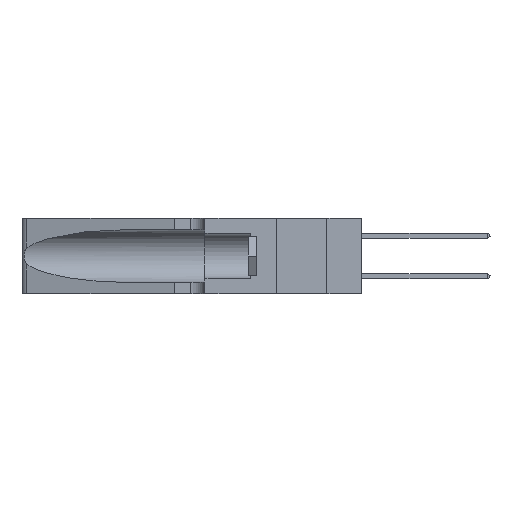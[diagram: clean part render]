
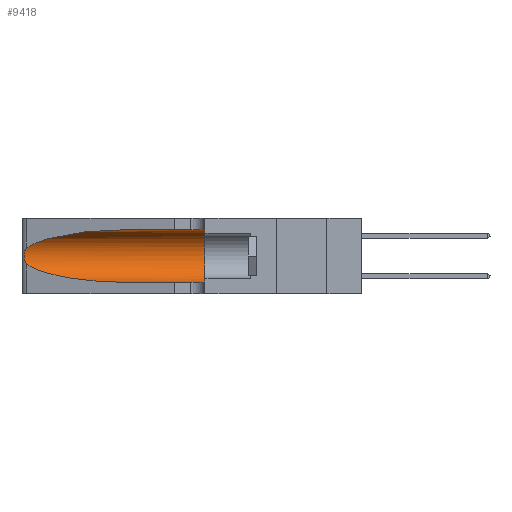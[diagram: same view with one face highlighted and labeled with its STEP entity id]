
A CAD part, left-side view. The second image highlights one B-rep face of the part: STEP entity #9418.
In plain terms, the highlighted cylindrical face has radius 3.308 mm (diameter 6.617 mm), a partial arc.
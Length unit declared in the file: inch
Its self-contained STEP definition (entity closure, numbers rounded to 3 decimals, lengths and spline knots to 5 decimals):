
#87 = LINE ( 'NONE', #23511, #12327 ) ;
#203 =( BOUNDED_CURVE ( )  B_SPLINE_CURVE ( 3, ( #25161, #13648, #16006, #1521 ),
 .UNSPECIFIED., .F., .F. ) 
 B_SPLINE_CURVE_WITH_KNOTS ( ( 4, 4 ),
 ( 3.44316, 4.71239 ),
 .UNSPECIFIED. ) 
 CURVE ( )  GEOMETRIC_REPRESENTATION_ITEM ( )  RATIONAL_B_SPLINE_CURVE ( ( 1., 0.87, 0.87, 1. ) ) 
 REPRESENTATION_ITEM ( '' )  );
#208 = CARTESIAN_POINT ( 'NONE',  ( 0.1305, 0.35, 0.31525 ) ) ;
#245 = CARTESIAN_POINT ( 'NONE',  ( 0.1305, 0.72297, 0.31525 ) ) ;
#1023 = CARTESIAN_POINT ( 'NONE',  ( 0.1305, 0.35, 0.185 ) ) ;
#1088 = CARTESIAN_POINT ( 'NONE',  ( 0.25787, 1.23484, 0.2124 ) ) ;
#1180 = B_SPLINE_CURVE_WITH_KNOTS ( 'NONE', 3,
 ( #27204, #29515, #15594, #1088, #17959, #3569, #20283, #6040, #22623, #8475, #24944, #10955, #27307, #13334 ),
 .UNSPECIFIED., .F., .F.,
 ( 4, 2, 2, 2, 2, 2, 4 ),
 ( 0., 0.00027, 0.00053, 0.00107, 0.0016, 0.00187, 0.00214 ),
 .UNSPECIFIED. ) ;
#1521 = CARTESIAN_POINT ( 'NONE',  ( 0.1305, 0.72297, 0.05475 ) ) ;
#1813 = EDGE_CURVE ( 'NONE', #19770, #26988, #3550, .T. ) ;
#2785 = ORIENTED_EDGE ( 'NONE', *, *, #14595, .T. ) ;
#3497 = DIRECTION ( 'NONE',  ( 0., 0., 1. ) ) ;
#3550 =( BOUNDED_CURVE ( )  B_SPLINE_CURVE ( 3, ( #245, #28720, #7532, #17137 ),
 .UNSPECIFIED., .F., .F. ) 
 B_SPLINE_CURVE_WITH_KNOTS ( ( 4, 4 ),
 ( 1.5708, 2.84003 ),
 .UNSPECIFIED. ) 
 CURVE ( )  GEOMETRIC_REPRESENTATION_ITEM ( )  RATIONAL_B_SPLINE_CURVE ( ( 1., 0.87, 0.87, 1. ) ) 
 REPRESENTATION_ITEM ( '' )  );
#3569 = CARTESIAN_POINT ( 'NONE',  ( 0.26018, 1.23835, 0.19895 ) ) ;
#3670 = EDGE_CURVE ( 'NONE', #19770, #26783, #16084, .T. ) ;
#5677 = CARTESIAN_POINT ( 'NONE',  ( 0.25487, 1.22718, 0.22369 ) ) ;
#6040 = CARTESIAN_POINT ( 'NONE',  ( 0.26075, 1.23896, 0.178 ) ) ;
#7050 = ORIENTED_EDGE ( 'NONE', *, *, #1813, .T. ) ;
#7532 = CARTESIAN_POINT ( 'NONE',  ( 0.2373, 1.15595, 0.28018 ) ) ;
#7551 = EDGE_CURVE ( 'NONE', #8156, #12607, #87, .T. ) ;
#8156 = VERTEX_POINT ( 'NONE', #30273 ) ;
#8475 = CARTESIAN_POINT ( 'NONE',  ( 0.25856, 1.23593, 0.16098 ) ) ;
#9418 = ADVANCED_FACE ( 'NONE', ( #23163 ), #22436, .F. ) ;
#9447 = DIRECTION ( 'NONE',  ( 0., -1., 0. ) ) ;
#9835 = ORIENTED_EDGE ( 'NONE', *, *, #19317, .T. ) ;
#10521 = VECTOR ( 'NONE', #18555, 39.37008 ) ;
#10955 = CARTESIAN_POINT ( 'NONE',  ( 0.25639, 1.23186, 0.15144 ) ) ;
#11575 = CARTESIAN_POINT ( 'NONE',  ( 0.1305, 1.61858, 0.185 ) ) ;
#11638 = CARTESIAN_POINT ( 'NONE',  ( 0.1305, 0.35, 0.05475 ) ) ;
#11726 = ORIENTED_EDGE ( 'NONE', *, *, #13005, .F. ) ;
#12327 = VECTOR ( 'NONE', #9447, 39.37008 ) ;
#12607 = VERTEX_POINT ( 'NONE', #11638 ) ;
#13005 = EDGE_CURVE ( 'NONE', #26783, #12607, #24573, .T. ) ;
#13021 = AXIS2_PLACEMENT_3D ( 'NONE', #1023, #17888, #3497 ) ;
#13334 = CARTESIAN_POINT ( 'NONE',  ( 0.25487, 1.22718, 0.14631 ) ) ;
#13648 = CARTESIAN_POINT ( 'NONE',  ( 0.2373, 1.15595, 0.08982 ) ) ;
#14595 = EDGE_CURVE ( 'NONE', #26988, #21667, #1180, .T. ) ;
#14648 = ORIENTED_EDGE ( 'NONE', *, *, #7551, .T. ) ;
#15192 = ORIENTED_EDGE ( 'NONE', *, *, #3670, .F. ) ;
#15594 = CARTESIAN_POINT ( 'NONE',  ( 0.25639, 1.23184, 0.21858 ) ) ;
#16006 = CARTESIAN_POINT ( 'NONE',  ( 0.18966, 0.96281, 0.05475 ) ) ;
#16084 = LINE ( 'NONE', #16227, #10521 ) ;
#16227 = CARTESIAN_POINT ( 'NONE',  ( 0.1305, 1.61858, 0.31525 ) ) ;
#16307 = DIRECTION ( 'NONE',  ( 0., -1., 0. ) ) ;
#17137 = CARTESIAN_POINT ( 'NONE',  ( 0.25487, 1.22718, 0.22369 ) ) ;
#17888 = DIRECTION ( 'NONE',  ( 0., 1., 0. ) ) ;
#17959 = CARTESIAN_POINT ( 'NONE',  ( 0.25854, 1.2359, 0.20912 ) ) ;
#18123 = AXIS2_PLACEMENT_3D ( 'NONE', #11575, #16307, #23222 ) ;
#18555 = DIRECTION ( 'NONE',  ( 0., -1., 0. ) ) ;
#19317 = EDGE_CURVE ( 'NONE', #21667, #8156, #203, .T. ) ;
#19770 = VERTEX_POINT ( 'NONE', #21535 ) ;
#20283 = CARTESIAN_POINT ( 'NONE',  ( 0.26075, 1.23896, 0.19203 ) ) ;
#21535 = CARTESIAN_POINT ( 'NONE',  ( 0.1305, 0.72297, 0.31525 ) ) ;
#21667 = VERTEX_POINT ( 'NONE', #28671 ) ;
#22436 = CYLINDRICAL_SURFACE ( 'NONE', #18123, 0.13025 ) ;
#22623 = CARTESIAN_POINT ( 'NONE',  ( 0.26017, 1.23833, 0.17102 ) ) ;
#23163 = FACE_OUTER_BOUND ( 'NONE', #26831, .T. ) ;
#23222 = DIRECTION ( 'NONE',  ( 0., 0., -1. ) ) ;
#23511 = CARTESIAN_POINT ( 'NONE',  ( 0.1305, 1.61858, 0.05475 ) ) ;
#24573 = CIRCLE ( 'NONE', #13021, 0.13025 ) ;
#24944 = CARTESIAN_POINT ( 'NONE',  ( 0.25789, 1.23486, 0.15765 ) ) ;
#25161 = CARTESIAN_POINT ( 'NONE',  ( 0.25487, 1.22718, 0.14631 ) ) ;
#26783 = VERTEX_POINT ( 'NONE', #208 ) ;
#26831 = EDGE_LOOP ( 'NONE', ( #7050, #2785, #9835, #14648, #11726, #15192 ) ) ;
#26988 = VERTEX_POINT ( 'NONE', #5677 ) ;
#27204 = CARTESIAN_POINT ( 'NONE',  ( 0.25487, 1.22718, 0.22369 ) ) ;
#27307 = CARTESIAN_POINT ( 'NONE',  ( 0.25555, 1.22993, 0.14849 ) ) ;
#28671 = CARTESIAN_POINT ( 'NONE',  ( 0.25487, 1.22718, 0.14631 ) ) ;
#28720 = CARTESIAN_POINT ( 'NONE',  ( 0.18966, 0.96281, 0.31525 ) ) ;
#29515 = CARTESIAN_POINT ( 'NONE',  ( 0.25555, 1.22994, 0.2215 ) ) ;
#30273 = CARTESIAN_POINT ( 'NONE',  ( 0.1305, 0.72297, 0.05475 ) ) ;
